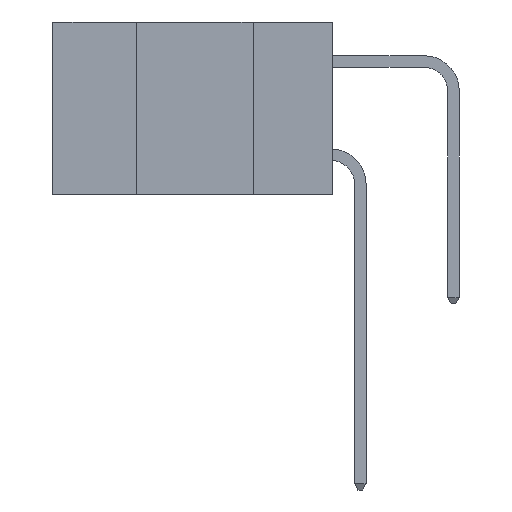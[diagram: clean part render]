
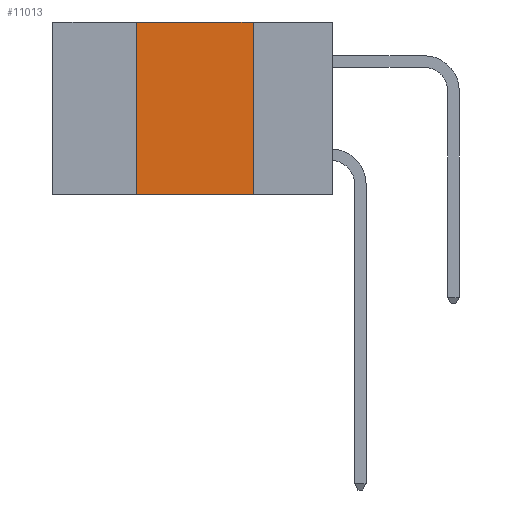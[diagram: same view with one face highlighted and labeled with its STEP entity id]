
A CAD part, left-side view. The second image highlights one B-rep face of the part: STEP entity #11013.
In plain terms, the highlighted planar face has unit normal (-1, 0, 0).
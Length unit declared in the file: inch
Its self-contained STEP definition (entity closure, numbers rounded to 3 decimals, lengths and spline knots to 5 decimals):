
#359 = CARTESIAN_POINT ( 'NONE',  ( 0., 0.42, -0.37 ) ) ;
#458 = LINE ( 'NONE', #13836, #11094 ) ;
#762 = ORIENTED_EDGE ( 'NONE', *, *, #11734, .F. ) ;
#953 = DIRECTION ( 'NONE',  ( 0., 0., 1. ) ) ;
#1410 = VECTOR ( 'NONE', #13724, 39.37008 ) ;
#1874 = ORIENTED_EDGE ( 'NONE', *, *, #9006, .T. ) ;
#3366 = CARTESIAN_POINT ( 'NONE',  ( 0., 0.6, 0. ) ) ;
#3493 = CARTESIAN_POINT ( 'NONE',  ( 0., 0.17, -0.37 ) ) ;
#3544 = CARTESIAN_POINT ( 'NONE',  ( 0., 0.42, 0. ) ) ;
#4019 = VERTEX_POINT ( 'NONE', #3544 ) ;
#4418 = CARTESIAN_POINT ( 'NONE',  ( 0., 0.6, 0. ) ) ;
#5505 = CARTESIAN_POINT ( 'NONE',  ( 0., 0.17, -0.37 ) ) ;
#6952 = PLANE ( 'NONE',  #11786 ) ;
#7199 = VECTOR ( 'NONE', #12858, 39.37008 ) ;
#7626 = EDGE_LOOP ( 'NONE', ( #762, #11928, #14793, #1874 ) ) ;
#7962 = LINE ( 'NONE', #8338, #10695 ) ;
#8124 = DIRECTION ( 'NONE',  ( 0., 0., -1. ) ) ;
#8239 = DIRECTION ( 'NONE',  ( 0., -1., 0. ) ) ;
#8338 = CARTESIAN_POINT ( 'NONE',  ( 0., 0.6, -0.37 ) ) ;
#9006 = EDGE_CURVE ( 'NONE', #10137, #12725, #7962, .T. ) ;
#10137 = VERTEX_POINT ( 'NONE', #359 ) ;
#10228 = VERTEX_POINT ( 'NONE', #11111 ) ;
#10653 = LINE ( 'NONE', #3493, #7199 ) ;
#10695 = VECTOR ( 'NONE', #8239, 39.37008 ) ;
#11013 = ADVANCED_FACE ( 'NONE', ( #11155 ), #6952, .F. ) ;
#11094 = VECTOR ( 'NONE', #953, 39.37008 ) ;
#11111 = CARTESIAN_POINT ( 'NONE',  ( 0., 0.17, 0. ) ) ;
#11155 = FACE_OUTER_BOUND ( 'NONE', #7626, .T. ) ;
#11734 = EDGE_CURVE ( 'NONE', #10228, #12725, #10653, .T. ) ;
#11786 = AXIS2_PLACEMENT_3D ( 'NONE', #3366, #15001, #8124 ) ;
#11928 = ORIENTED_EDGE ( 'NONE', *, *, #12807, .F. ) ;
#12725 = VERTEX_POINT ( 'NONE', #5505 ) ;
#12807 = EDGE_CURVE ( 'NONE', #4019, #10228, #13847, .T. ) ;
#12858 = DIRECTION ( 'NONE',  ( 0., 0., -1. ) ) ;
#13724 = DIRECTION ( 'NONE',  ( 0., -1., 0. ) ) ;
#13836 = CARTESIAN_POINT ( 'NONE',  ( 0., 0.42, -0.37 ) ) ;
#13847 = LINE ( 'NONE', #4418, #1410 ) ;
#14103 = EDGE_CURVE ( 'NONE', #10137, #4019, #458, .T. ) ;
#14793 = ORIENTED_EDGE ( 'NONE', *, *, #14103, .F. ) ;
#15001 = DIRECTION ( 'NONE',  ( 1., 0., 0. ) ) ;
